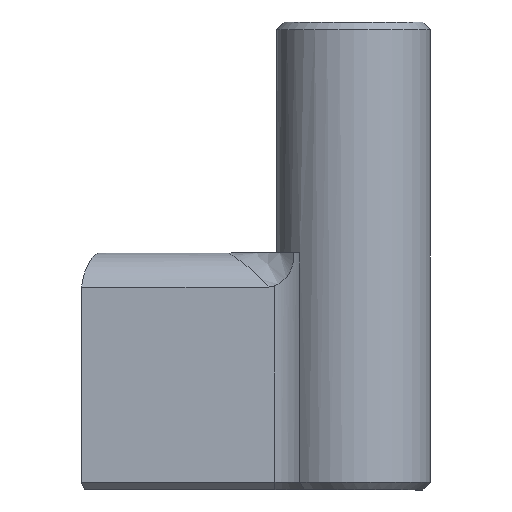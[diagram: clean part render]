
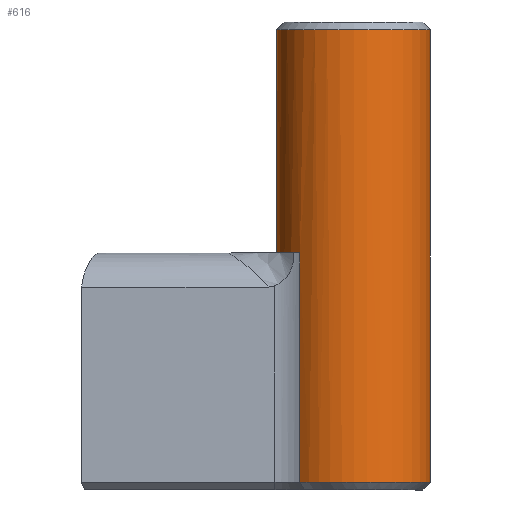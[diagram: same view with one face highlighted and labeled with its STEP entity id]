
A CAD part, front view. The second image highlights one B-rep face of the part: STEP entity #616.
In plain terms, the highlighted cylindrical face has radius 5.1 mm (diameter 10.2 mm), a full revolution.
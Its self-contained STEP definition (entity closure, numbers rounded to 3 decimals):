
#21=CYLINDRICAL_SURFACE('',#685,5.1);
#76=LINE('',#1086,#114);
#77=LINE('',#1088,#115);
#78=LINE('',#1091,#116);
#114=VECTOR('',#799,5.1);
#115=VECTOR('',#800,10.);
#116=VECTOR('',#803,10.);
#149=FACE_OUTER_BOUND('',#188,.T.);
#188=EDGE_LOOP('',(#473,#474,#475,#476,#477,#478,#479,#480,#481));
#241=CIRCLE('',#661,5.1);
#242=CIRCLE('',#662,5.1);
#248=CIRCLE('',#681,5.1);
#249=CIRCLE('',#682,5.1);
#251=CIRCLE('',#686,5.1);
#265=VERTEX_POINT('',#896);
#266=VERTEX_POINT('',#904);
#267=VERTEX_POINT('',#906);
#294=VERTEX_POINT('',#1077);
#295=VERTEX_POINT('',#1079);
#297=VERTEX_POINT('',#1087);
#298=VERTEX_POINT('',#1089);
#324=EDGE_CURVE('',#265,#266,#241,.T.);
#325=EDGE_CURVE('',#266,#267,#242,.T.);
#361=EDGE_CURVE('',#294,#295,#248,.T.);
#362=EDGE_CURVE('',#295,#294,#249,.T.);
#364=EDGE_CURVE('',#295,#266,#76,.T.);
#365=EDGE_CURVE('',#265,#297,#77,.T.);
#366=EDGE_CURVE('',#297,#298,#251,.T.);
#367=EDGE_CURVE('',#267,#298,#78,.T.);
#473=ORIENTED_EDGE('',*,*,#361,.F.);
#474=ORIENTED_EDGE('',*,*,#362,.F.);
#475=ORIENTED_EDGE('',*,*,#364,.T.);
#476=ORIENTED_EDGE('',*,*,#324,.F.);
#477=ORIENTED_EDGE('',*,*,#365,.T.);
#478=ORIENTED_EDGE('',*,*,#366,.T.);
#479=ORIENTED_EDGE('',*,*,#367,.F.);
#480=ORIENTED_EDGE('',*,*,#325,.F.);
#481=ORIENTED_EDGE('',*,*,#364,.F.);
#616=ADVANCED_FACE('',(#149),#21,.T.);
#661=AXIS2_PLACEMENT_3D('',#905,#730,#731);
#662=AXIS2_PLACEMENT_3D('',#907,#732,#733);
#681=AXIS2_PLACEMENT_3D('',#1080,#789,#790);
#682=AXIS2_PLACEMENT_3D('',#1081,#791,#792);
#685=AXIS2_PLACEMENT_3D('',#1085,#797,#798);
#686=AXIS2_PLACEMENT_3D('',#1090,#801,#802);
#730=DIRECTION('center_axis',(0.,0.,
-1.));
#731=DIRECTION('ref_axis',(0.,-1.,0.));
#732=DIRECTION('center_axis',(0.,0.,
-1.));
#733=DIRECTION('ref_axis',(0.,-1.,0.));
#789=DIRECTION('center_axis',(0.,0.,
1.));
#790=DIRECTION('ref_axis',(0.,-1.,0.));
#791=DIRECTION('center_axis',(0.,0.,
1.));
#792=DIRECTION('ref_axis',(0.,-1.,0.));
#797=DIRECTION('center_axis',(0.,0.,
1.));
#798=DIRECTION('ref_axis',(0.,1.,0.));
#799=DIRECTION('',(0.,0.,-1.));
#800=DIRECTION('',(0.,0.,1.));
#801=DIRECTION('center_axis',(0.,0.,
1.));
#802=DIRECTION('ref_axis',(0.,-1.,0.));
#803=DIRECTION('',(0.,0.,1.));
#896=CARTESIAN_POINT('',(130.892,209.985,-53.067));
#904=CARTESIAN_POINT('',(132.472,200.036,-53.067));
#905=CARTESIAN_POINT('Origin',(132.472,205.136,-53.067));
#906=CARTESIAN_POINT('',(128.922,201.474,-53.067));
#907=CARTESIAN_POINT('Origin',(132.472,205.136,-53.067));
#1077=CARTESIAN_POINT('',(132.472,210.236,-23.067));
#1079=CARTESIAN_POINT('',(132.472,200.036,-23.067));
#1080=CARTESIAN_POINT('Origin',(132.472,205.136,-23.067));
#1081=CARTESIAN_POINT('Origin',(132.472,205.136,-23.067));
#1085=CARTESIAN_POINT('Origin',(132.472,205.136,-53.567));
#1086=CARTESIAN_POINT('',(132.472,200.036,-53.567));
#1087=CARTESIAN_POINT('',(130.892,209.985,-37.867));
#1088=CARTESIAN_POINT('',(130.892,209.985,-53.567));
#1089=CARTESIAN_POINT('',(128.922,201.474,-37.867));
#1090=CARTESIAN_POINT('Origin',(132.472,205.136,-37.867));
#1091=CARTESIAN_POINT('',(128.922,201.474,-53.567));
